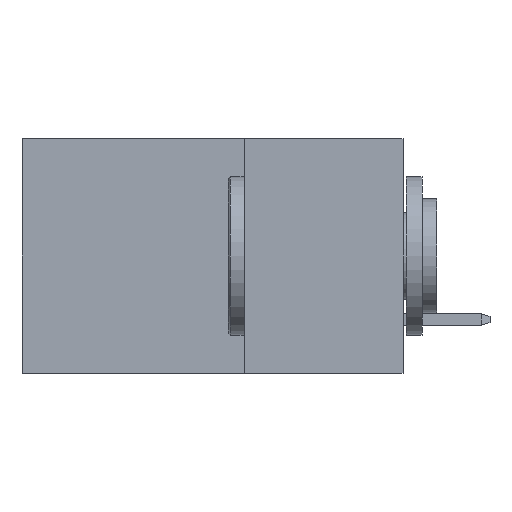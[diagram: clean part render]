
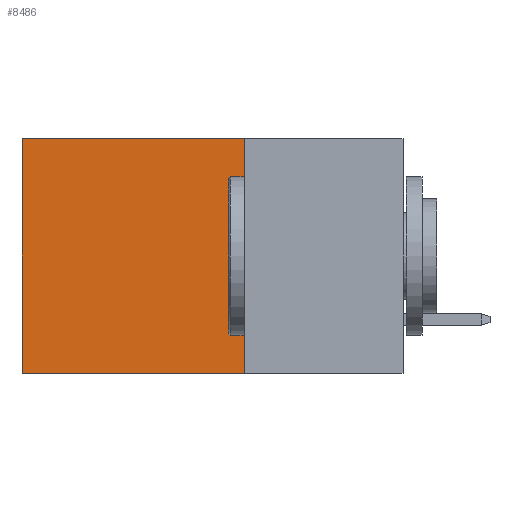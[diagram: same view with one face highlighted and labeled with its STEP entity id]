
A CAD part, left-side view. The second image highlights one B-rep face of the part: STEP entity #8486.
In plain terms, the highlighted planar face has unit normal (-1, 0, 0).
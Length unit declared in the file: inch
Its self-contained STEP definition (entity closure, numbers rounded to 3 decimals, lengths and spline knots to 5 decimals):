
#614 = CARTESIAN_POINT ( 'NONE',  ( 0.2875, 0.6, 0. ) ) ;
#1597 = LINE ( 'NONE', #14399, #11632 ) ;
#2162 = LINE ( 'NONE', #6968, #10035 ) ;
#2425 = CARTESIAN_POINT ( 'NONE',  ( 0.2875, 0.25, 0. ) ) ;
#2854 = VECTOR ( 'NONE', #6048, 39.37008 ) ;
#3296 = VERTEX_POINT ( 'NONE', #614 ) ;
#3502 = EDGE_LOOP ( 'NONE', ( #8044, #8721, #7761, #7756 ) ) ;
#3539 = DIRECTION ( 'NONE',  ( 0., 0., -1. ) ) ;
#3634 = VERTEX_POINT ( 'NONE', #10495 ) ;
#3671 = DIRECTION ( 'NONE',  ( 0., 1., 0. ) ) ;
#4392 = VERTEX_POINT ( 'NONE', #6522 ) ;
#4463 = CARTESIAN_POINT ( 'NONE',  ( 0.2875, 0.25, 0. ) ) ;
#4594 = EDGE_CURVE ( 'NONE', #3634, #4392, #7694, .T. ) ;
#4728 = PLANE ( 'NONE',  #7165 ) ;
#6048 = DIRECTION ( 'NONE',  ( 0., 0., -1. ) ) ;
#6322 = EDGE_CURVE ( 'NONE', #3296, #12043, #2162, .T. ) ;
#6354 = EDGE_CURVE ( 'NONE', #3634, #3296, #10249, .T. ) ;
#6522 = CARTESIAN_POINT ( 'NONE',  ( 0.2875, 0.25, -0.37 ) ) ;
#6968 = CARTESIAN_POINT ( 'NONE',  ( 0.2875, 0.6, 0. ) ) ;
#7165 = AXIS2_PLACEMENT_3D ( 'NONE', #2425, #9595, #13014 ) ;
#7694 = LINE ( 'NONE', #13118, #2854 ) ;
#7756 = ORIENTED_EDGE ( 'NONE', *, *, #6354, .T. ) ;
#7761 = ORIENTED_EDGE ( 'NONE', *, *, #4594, .F. ) ;
#8044 = ORIENTED_EDGE ( 'NONE', *, *, #6322, .T. ) ;
#8486 = ADVANCED_FACE ( 'NONE', ( #9518 ), #4728, .F. ) ;
#8721 = ORIENTED_EDGE ( 'NONE', *, *, #14036, .F. ) ;
#9518 = FACE_OUTER_BOUND ( 'NONE', #3502, .T. ) ;
#9595 = DIRECTION ( 'NONE',  ( 1., 0., 0. ) ) ;
#10035 = VECTOR ( 'NONE', #3539, 39.37008 ) ;
#10249 = LINE ( 'NONE', #4463, #12707 ) ;
#10318 = DIRECTION ( 'NONE',  ( 0., 1., 0. ) ) ;
#10495 = CARTESIAN_POINT ( 'NONE',  ( 0.2875, 0.25, 0. ) ) ;
#11632 = VECTOR ( 'NONE', #3671, 39.37008 ) ;
#12043 = VERTEX_POINT ( 'NONE', #13513 ) ;
#12707 = VECTOR ( 'NONE', #10318, 39.37008 ) ;
#13014 = DIRECTION ( 'NONE',  ( 0., 0., -1. ) ) ;
#13118 = CARTESIAN_POINT ( 'NONE',  ( 0.2875, 0.25, 0. ) ) ;
#13513 = CARTESIAN_POINT ( 'NONE',  ( 0.2875, 0.6, -0.37 ) ) ;
#14036 = EDGE_CURVE ( 'NONE', #4392, #12043, #1597, .T. ) ;
#14399 = CARTESIAN_POINT ( 'NONE',  ( 0.2875, 0.25, -0.37 ) ) ;
